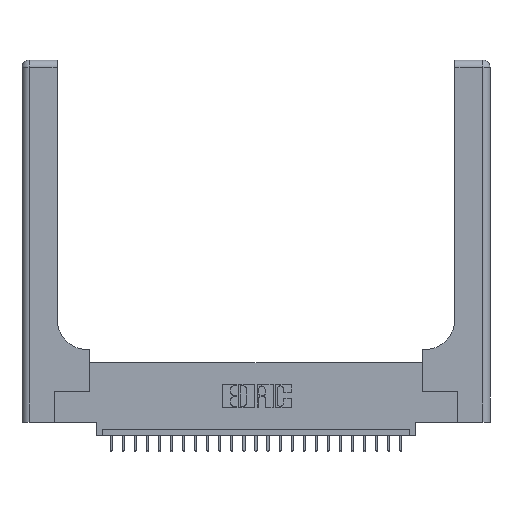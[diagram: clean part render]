
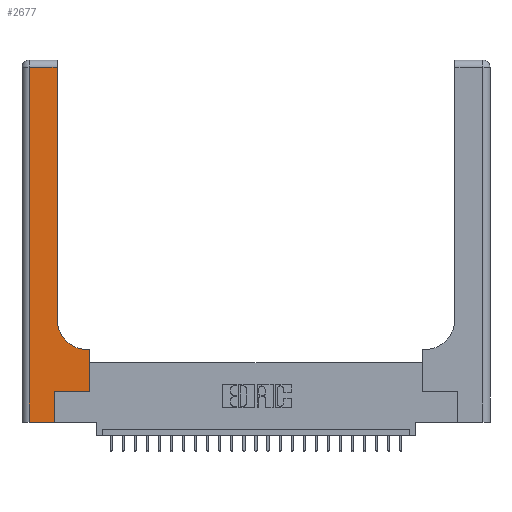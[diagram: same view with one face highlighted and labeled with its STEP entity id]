
A CAD part, top view. The second image highlights one B-rep face of the part: STEP entity #2677.
In plain terms, the highlighted planar face has unit normal (0, 0, 1).
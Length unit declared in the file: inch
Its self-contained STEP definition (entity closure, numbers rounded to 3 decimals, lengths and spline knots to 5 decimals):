
#345 = VECTOR ( 'NONE', #25292, 39.37008 ) ;
#489 = DIRECTION ( 'NONE',  ( 0., 1., 0. ) ) ;
#950 = PLANE ( 'NONE',  #17482 ) ;
#984 = VERTEX_POINT ( 'NONE', #9220 ) ;
#1828 = VECTOR ( 'NONE', #16195, 39.37008 ) ;
#2677 = ADVANCED_FACE ( 'NONE', ( #13482 ), #950, .F. ) ;
#3069 = VERTEX_POINT ( 'NONE', #20081 ) ;
#3302 = EDGE_CURVE ( 'NONE', #13117, #26126, #5590, .T. ) ;
#3623 = EDGE_LOOP ( 'NONE', ( #25200, #25252, #3696, #11035, #16007, #19378, #21147, #14469, #18819 ) ) ;
#3644 = CARTESIAN_POINT ( 'NONE',  ( 0.5415, 0.6, 0.37 ) ) ;
#3696 = ORIENTED_EDGE ( 'NONE', *, *, #7933, .T. ) ;
#4014 = CARTESIAN_POINT ( 'NONE',  ( 0.06, 2.94, 0.37 ) ) ;
#5370 = VECTOR ( 'NONE', #17227, 39.37008 ) ;
#5590 = LINE ( 'NONE', #11760, #11949 ) ;
#5976 = LINE ( 'NONE', #16433, #12064 ) ;
#6237 = LINE ( 'NONE', #14424, #20095 ) ;
#6542 = CARTESIAN_POINT ( 'NONE',  ( 0., 0., 0.37 ) ) ;
#6618 = VERTEX_POINT ( 'NONE', #4014 ) ;
#7016 = CIRCLE ( 'NONE', #8794, 0.25 ) ;
#7768 = EDGE_CURVE ( 'NONE', #16775, #3069, #7016, .T. ) ;
#7933 = EDGE_CURVE ( 'NONE', #6618, #10225, #9197, .T. ) ;
#8018 = CARTESIAN_POINT ( 'NONE',  ( 0.2915, 3., 0.37 ) ) ;
#8161 = LINE ( 'NONE', #8018, #1828 ) ;
#8284 = CARTESIAN_POINT ( 'NONE',  ( 0.5415, 0.85, 0.37 ) ) ;
#8794 = AXIS2_PLACEMENT_3D ( 'NONE', #8284, #10518, #10137 ) ;
#9027 = DIRECTION ( 'NONE',  ( -1., 0., 0. ) ) ;
#9197 = LINE ( 'NONE', #25486, #5370 ) ;
#9220 = CARTESIAN_POINT ( 'NONE',  ( 0.269, 0.25, 0.37 ) ) ;
#10137 = DIRECTION ( 'NONE',  ( 1., 0., 0. ) ) ;
#10225 = VERTEX_POINT ( 'NONE', #13165 ) ;
#10518 = DIRECTION ( 'NONE',  ( 0., 0., -1. ) ) ;
#10708 = LINE ( 'NONE', #18884, #345 ) ;
#10925 = CARTESIAN_POINT ( 'NONE',  ( 0.269, 0., 0.37 ) ) ;
#11035 = ORIENTED_EDGE ( 'NONE', *, *, #24477, .T. ) ;
#11760 = CARTESIAN_POINT ( 'NONE',  ( 0.5585, 0.25, 0.37 ) ) ;
#11949 = VECTOR ( 'NONE', #21499, 39.37008 ) ;
#12064 = VECTOR ( 'NONE', #20793, 39.37008 ) ;
#12481 = VERTEX_POINT ( 'NONE', #10925 ) ;
#12616 = LINE ( 'NONE', #20728, #23922 ) ;
#13117 = VERTEX_POINT ( 'NONE', #16760 ) ;
#13165 = CARTESIAN_POINT ( 'NONE',  ( 0.06, 0., 0.37 ) ) ;
#13482 = FACE_OUTER_BOUND ( 'NONE', #3623, .T. ) ;
#14424 = CARTESIAN_POINT ( 'NONE',  ( 0.269, 0.25, 0.37 ) ) ;
#14469 = ORIENTED_EDGE ( 'NONE', *, *, #23217, .T. ) ;
#14746 = DIRECTION ( 'NONE',  ( 1., 0., 0. ) ) ;
#16007 = ORIENTED_EDGE ( 'NONE', *, *, #24311, .T. ) ;
#16195 = DIRECTION ( 'NONE',  ( 0., 1., 0. ) ) ;
#16433 = CARTESIAN_POINT ( 'NONE',  ( 0., 2.94, 0.37 ) ) ;
#16760 = CARTESIAN_POINT ( 'NONE',  ( 0.5585, 0.25, 0.37 ) ) ;
#16775 = VERTEX_POINT ( 'NONE', #3644 ) ;
#17227 = DIRECTION ( 'NONE',  ( 0., -1., 0. ) ) ;
#17482 = AXIS2_PLACEMENT_3D ( 'NONE', #25454, #19593, #9027 ) ;
#17499 = EDGE_CURVE ( 'NONE', #20716, #6618, #5976, .T. ) ;
#18819 = ORIENTED_EDGE ( 'NONE', *, *, #7768, .T. ) ;
#18884 = CARTESIAN_POINT ( 'NONE',  ( 0.2915, 0.6, 0.37 ) ) ;
#19199 = CARTESIAN_POINT ( 'NONE',  ( 0.2915, 2.94, 0.37 ) ) ;
#19269 = VECTOR ( 'NONE', #14746, 39.37008 ) ;
#19378 = ORIENTED_EDGE ( 'NONE', *, *, #23855, .T. ) ;
#19593 = DIRECTION ( 'NONE',  ( 0., 0., -1. ) ) ;
#19663 = EDGE_CURVE ( 'NONE', #3069, #20716, #8161, .T. ) ;
#19872 = CARTESIAN_POINT ( 'NONE',  ( 0.5585, 0.6, 0.37 ) ) ;
#20081 = CARTESIAN_POINT ( 'NONE',  ( 0.2915, 0.85, 0.37 ) ) ;
#20095 = VECTOR ( 'NONE', #22523, 39.37008 ) ;
#20432 = LINE ( 'NONE', #6542, #19269 ) ;
#20716 = VERTEX_POINT ( 'NONE', #19199 ) ;
#20728 = CARTESIAN_POINT ( 'NONE',  ( 0.269, 0., 0.37 ) ) ;
#20793 = DIRECTION ( 'NONE',  ( -1., 0., 0. ) ) ;
#21147 = ORIENTED_EDGE ( 'NONE', *, *, #3302, .T. ) ;
#21499 = DIRECTION ( 'NONE',  ( 0., 1., 0. ) ) ;
#22523 = DIRECTION ( 'NONE',  ( 1., 0., 0. ) ) ;
#23217 = EDGE_CURVE ( 'NONE', #26126, #16775, #10708, .T. ) ;
#23855 = EDGE_CURVE ( 'NONE', #984, #13117, #6237, .T. ) ;
#23922 = VECTOR ( 'NONE', #489, 39.37008 ) ;
#24311 = EDGE_CURVE ( 'NONE', #12481, #984, #12616, .T. ) ;
#24477 = EDGE_CURVE ( 'NONE', #10225, #12481, #20432, .T. ) ;
#25200 = ORIENTED_EDGE ( 'NONE', *, *, #19663, .T. ) ;
#25252 = ORIENTED_EDGE ( 'NONE', *, *, #17499, .T. ) ;
#25292 = DIRECTION ( 'NONE',  ( -1., 0., 0. ) ) ;
#25454 = CARTESIAN_POINT ( 'NONE',  ( 0., 3., 0.37 ) ) ;
#25486 = CARTESIAN_POINT ( 'NONE',  ( 0.06, 3., 0.37 ) ) ;
#26126 = VERTEX_POINT ( 'NONE', #19872 ) ;
